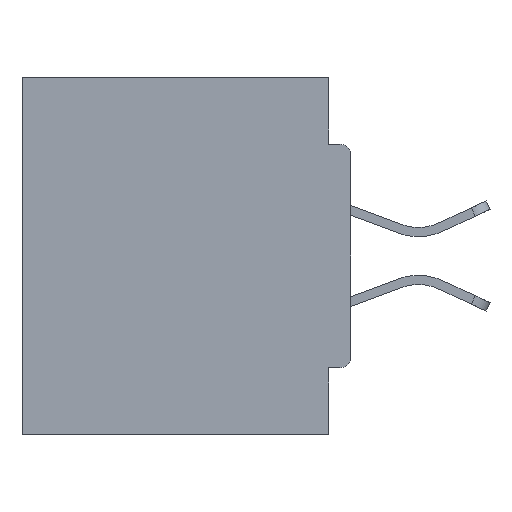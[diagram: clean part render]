
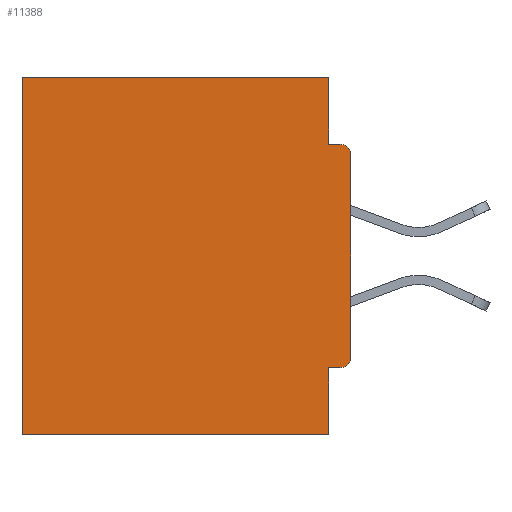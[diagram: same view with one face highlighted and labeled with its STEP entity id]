
A CAD part, left-side view. The second image highlights one B-rep face of the part: STEP entity #11388.
In plain terms, the highlighted planar face has unit normal (-1, 0, 0).
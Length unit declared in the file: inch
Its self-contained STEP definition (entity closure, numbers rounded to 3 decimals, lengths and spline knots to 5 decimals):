
#846 = VECTOR ( 'NONE', #19590, 39.37008 ) ;
#989 = DIRECTION ( 'NONE',  ( 0., 0., -1. ) ) ;
#1213 = CARTESIAN_POINT ( 'NONE',  ( 0.298, 0.031, -0.5 ) ) ;
#1314 = VERTEX_POINT ( 'NONE', #15490 ) ;
#1576 = ORIENTED_EDGE ( 'NONE', *, *, #15912, .F. ) ;
#1705 = DIRECTION ( 'NONE',  ( -1., 0., 0. ) ) ;
#1932 = CARTESIAN_POINT ( 'NONE',  ( 0.298, 0.015, -0.3915 ) ) ;
#2500 = DIRECTION ( 'NONE',  ( 0., 1., 0. ) ) ;
#3744 = CARTESIAN_POINT ( 'NONE',  ( 0.298, 0.46, 0. ) ) ;
#4939 = LINE ( 'NONE', #31303, #25008 ) ;
#5166 = AXIS2_PLACEMENT_3D ( 'NONE', #21888, #29550, #13870 ) ;
#5615 = DIRECTION ( 'NONE',  ( 0., 0., -1. ) ) ;
#5641 = VECTOR ( 'NONE', #2500, 39.37008 ) ;
#5775 = DIRECTION ( 'NONE',  ( 0., 1., 0. ) ) ;
#5842 = ORIENTED_EDGE ( 'NONE', *, *, #15959, .T. ) ;
#6141 = VERTEX_POINT ( 'NONE', #19531 ) ;
#6697 = ORIENTED_EDGE ( 'NONE', *, *, #19087, .F. ) ;
#6821 = EDGE_LOOP ( 'NONE', ( #5842, #30832, #8564, #32801, #11788, #6697, #1576, #7705, #11414, #11687 ) ) ;
#7268 = CARTESIAN_POINT ( 'NONE',  ( 0.298, 0.015, -0.4065 ) ) ;
#7457 = VECTOR ( 'NONE', #11703, 39.37008 ) ;
#7681 = LINE ( 'NONE', #15515, #5641 ) ;
#7705 = ORIENTED_EDGE ( 'NONE', *, *, #24578, .F. ) ;
#7713 = LINE ( 'NONE', #1213, #846 ) ;
#8231 = VERTEX_POINT ( 'NONE', #3744 ) ;
#8564 = ORIENTED_EDGE ( 'NONE', *, *, #21565, .F. ) ;
#8917 = DIRECTION ( 'NONE',  ( -1., 0., 0. ) ) ;
#9816 = VECTOR ( 'NONE', #5615, 39.37008 ) ;
#10322 = DIRECTION ( 'NONE',  ( 0., -1., 0. ) ) ;
#10340 = LINE ( 'NONE', #16207, #30395 ) ;
#10381 = EDGE_CURVE ( 'NONE', #8231, #29571, #15392, .T. ) ;
#11184 = CARTESIAN_POINT ( 'NONE',  ( 0.298, 0.46, -0.5 ) ) ;
#11351 = EDGE_CURVE ( 'NONE', #26656, #28228, #18179, .T. ) ;
#11388 = ADVANCED_FACE ( 'NONE', ( #28359 ), #29192, .F. ) ;
#11414 = ORIENTED_EDGE ( 'NONE', *, *, #24764, .T. ) ;
#11687 = ORIENTED_EDGE ( 'NONE', *, *, #26695, .F. ) ;
#11703 = DIRECTION ( 'NONE',  ( 0., 1., 0. ) ) ;
#11788 = ORIENTED_EDGE ( 'NONE', *, *, #10381, .T. ) ;
#13409 = CARTESIAN_POINT ( 'NONE',  ( 0.298, 0.015, -0.0935 ) ) ;
#13870 = DIRECTION ( 'NONE',  ( 0., 0., -1. ) ) ;
#14196 = VERTEX_POINT ( 'NONE', #7268 ) ;
#15392 = LINE ( 'NONE', #20959, #31351 ) ;
#15490 = CARTESIAN_POINT ( 'NONE',  ( 0.298, 0., -0.3915 ) ) ;
#15515 = CARTESIAN_POINT ( 'NONE',  ( 0.298, 0., 0. ) ) ;
#15821 = CARTESIAN_POINT ( 'NONE',  ( 0.298, 0., -0.0935 ) ) ;
#15912 = EDGE_CURVE ( 'NONE', #24091, #22598, #7713, .T. ) ;
#15946 = CARTESIAN_POINT ( 'NONE',  ( 0.298, 0., 0. ) ) ;
#15959 = EDGE_CURVE ( 'NONE', #19186, #28228, #22875, .T. ) ;
#16207 = CARTESIAN_POINT ( 'NONE',  ( 0.298, 0., -0.4065 ) ) ;
#16616 = CARTESIAN_POINT ( 'NONE',  ( 0.298, 0.015, -0.1085 ) ) ;
#18179 = LINE ( 'NONE', #15821, #24304 ) ;
#18792 = LINE ( 'NONE', #15946, #9816 ) ;
#19087 = EDGE_CURVE ( 'NONE', #22598, #29571, #26731, .T. ) ;
#19186 = VERTEX_POINT ( 'NONE', #20048 ) ;
#19531 = CARTESIAN_POINT ( 'NONE',  ( 0.298, 0.031, 0. ) ) ;
#19557 = CARTESIAN_POINT ( 'NONE',  ( 0.298, 0.031, -0.5 ) ) ;
#19590 = DIRECTION ( 'NONE',  ( 0., 0., -1. ) ) ;
#19726 = AXIS2_PLACEMENT_3D ( 'NONE', #1932, #1705, #20201 ) ;
#20048 = CARTESIAN_POINT ( 'NONE',  ( 0.298, 0., -0.1085 ) ) ;
#20201 = DIRECTION ( 'NONE',  ( 0., 0., -1. ) ) ;
#20959 = CARTESIAN_POINT ( 'NONE',  ( 0.298, 0.46, 0. ) ) ;
#21048 = AXIS2_PLACEMENT_3D ( 'NONE', #16616, #8917, #989 ) ;
#21565 = EDGE_CURVE ( 'NONE', #6141, #26656, #4939, .T. ) ;
#21888 = CARTESIAN_POINT ( 'NONE',  ( 0.298, 0., 0. ) ) ;
#22598 = VERTEX_POINT ( 'NONE', #19557 ) ;
#22875 = CIRCLE ( 'NONE', #21048, 0.015 ) ;
#24091 = VERTEX_POINT ( 'NONE', #30728 ) ;
#24304 = VECTOR ( 'NONE', #10322, 39.37008 ) ;
#24578 = EDGE_CURVE ( 'NONE', #14196, #24091, #10340, .T. ) ;
#24764 = EDGE_CURVE ( 'NONE', #14196, #1314, #33690, .T. ) ;
#25008 = VECTOR ( 'NONE', #26838, 39.37008 ) ;
#26254 = DIRECTION ( 'NONE',  ( 0., 0., -1. ) ) ;
#26656 = VERTEX_POINT ( 'NONE', #28749 ) ;
#26695 = EDGE_CURVE ( 'NONE', #19186, #1314, #18792, .T. ) ;
#26731 = LINE ( 'NONE', #30117, #7457 ) ;
#26838 = DIRECTION ( 'NONE',  ( 0., 0., -1. ) ) ;
#28228 = VERTEX_POINT ( 'NONE', #13409 ) ;
#28359 = FACE_OUTER_BOUND ( 'NONE', #6821, .T. ) ;
#28749 = CARTESIAN_POINT ( 'NONE',  ( 0.298, 0.031, -0.0935 ) ) ;
#29192 = PLANE ( 'NONE',  #5166 ) ;
#29550 = DIRECTION ( 'NONE',  ( 1., 0., 0. ) ) ;
#29571 = VERTEX_POINT ( 'NONE', #11184 ) ;
#30117 = CARTESIAN_POINT ( 'NONE',  ( 0.298, 0., -0.5 ) ) ;
#30395 = VECTOR ( 'NONE', #5775, 39.37008 ) ;
#30728 = CARTESIAN_POINT ( 'NONE',  ( 0.298, 0.031, -0.4065 ) ) ;
#30832 = ORIENTED_EDGE ( 'NONE', *, *, #11351, .F. ) ;
#31303 = CARTESIAN_POINT ( 'NONE',  ( 0.298, 0.031, -0.5 ) ) ;
#31351 = VECTOR ( 'NONE', #26254, 39.37008 ) ;
#32801 = ORIENTED_EDGE ( 'NONE', *, *, #33497, .T. ) ;
#33497 = EDGE_CURVE ( 'NONE', #6141, #8231, #7681, .T. ) ;
#33690 = CIRCLE ( 'NONE', #19726, 0.015 ) ;
